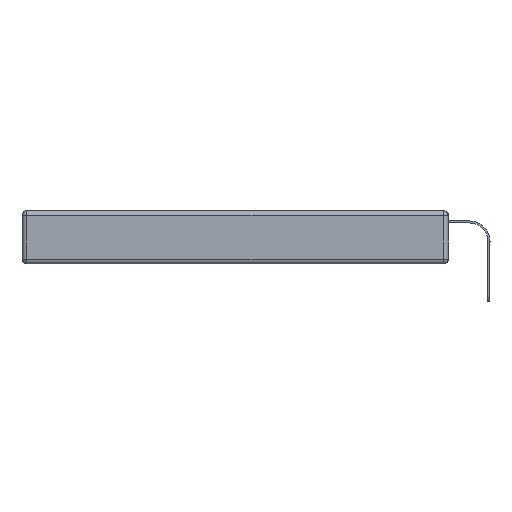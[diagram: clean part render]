
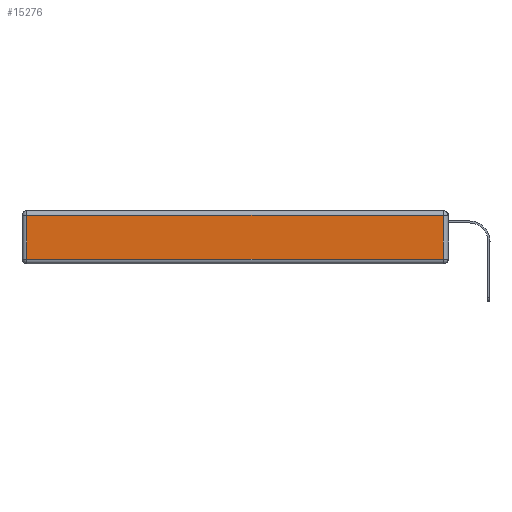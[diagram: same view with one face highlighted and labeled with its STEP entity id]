
A CAD part, left-side view. The second image highlights one B-rep face of the part: STEP entity #15276.
In plain terms, the highlighted planar face has unit normal (-1, 0, 0).
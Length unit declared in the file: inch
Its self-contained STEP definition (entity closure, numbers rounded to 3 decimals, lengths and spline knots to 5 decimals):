
#417 = DIRECTION ( 'NONE',  ( 0., 1., 0. ) ) ;
#748 = DIRECTION ( 'NONE',  ( 0., 0., -1. ) ) ;
#802 = VERTEX_POINT ( 'NONE', #14927 ) ;
#2166 = CARTESIAN_POINT ( 'NONE',  ( 0., 2.72, -0.343 ) ) ;
#2564 = VERTEX_POINT ( 'NONE', #5466 ) ;
#2790 = PLANE ( 'NONE',  #6405 ) ;
#4014 = VECTOR ( 'NONE', #417, 39.37008 ) ;
#4030 = DIRECTION ( 'NONE',  ( -1., 0., 0. ) ) ;
#4490 = EDGE_CURVE ( 'NONE', #13970, #2564, #10961, .T. ) ;
#4779 = DIRECTION ( 'NONE',  ( 0., 0., 1. ) ) ;
#5285 = CARTESIAN_POINT ( 'NONE',  ( 0., 2.72, -0.313 ) ) ;
#5466 = CARTESIAN_POINT ( 'NONE',  ( 0., 0.03, -0.313 ) ) ;
#6267 = LINE ( 'NONE', #2166, #12860 ) ;
#6405 = AXIS2_PLACEMENT_3D ( 'NONE', #16330, #4030, #16239 ) ;
#7189 = VERTEX_POINT ( 'NONE', #10764 ) ;
#7511 = ORIENTED_EDGE ( 'NONE', *, *, #17311, .T. ) ;
#8336 = EDGE_LOOP ( 'NONE', ( #15987, #7511, #16003, #10763 ) ) ;
#8865 = LINE ( 'NONE', #14305, #11565 ) ;
#10025 = CARTESIAN_POINT ( 'NONE',  ( 0., 2.75, -0.03 ) ) ;
#10682 = EDGE_CURVE ( 'NONE', #802, #7189, #14222, .T. ) ;
#10763 = ORIENTED_EDGE ( 'NONE', *, *, #12595, .T. ) ;
#10764 = CARTESIAN_POINT ( 'NONE',  ( 0., 2.72, -0.03 ) ) ;
#10800 = FACE_OUTER_BOUND ( 'NONE', #8336, .T. ) ;
#10961 = LINE ( 'NONE', #16402, #16889 ) ;
#11565 = VECTOR ( 'NONE', #4779, 39.37008 ) ;
#12031 = DIRECTION ( 'NONE',  ( 0., -1., 0. ) ) ;
#12595 = EDGE_CURVE ( 'NONE', #7189, #13970, #6267, .T. ) ;
#12860 = VECTOR ( 'NONE', #748, 39.37008 ) ;
#13970 = VERTEX_POINT ( 'NONE', #5285 ) ;
#14222 = LINE ( 'NONE', #10025, #4014 ) ;
#14305 = CARTESIAN_POINT ( 'NONE',  ( 0., 0.03, -0.343 ) ) ;
#14927 = CARTESIAN_POINT ( 'NONE',  ( 0., 0.03, -0.03 ) ) ;
#15276 = ADVANCED_FACE ( 'NONE', ( #10800 ), #2790, .T. ) ;
#15987 = ORIENTED_EDGE ( 'NONE', *, *, #4490, .T. ) ;
#16003 = ORIENTED_EDGE ( 'NONE', *, *, #10682, .T. ) ;
#16239 = DIRECTION ( 'NONE',  ( 0., 0., 1. ) ) ;
#16330 = CARTESIAN_POINT ( 'NONE',  ( 0., 0., -0.343 ) ) ;
#16402 = CARTESIAN_POINT ( 'NONE',  ( 0., 0., -0.313 ) ) ;
#16889 = VECTOR ( 'NONE', #12031, 39.37008 ) ;
#17311 = EDGE_CURVE ( 'NONE', #2564, #802, #8865, .T. ) ;
